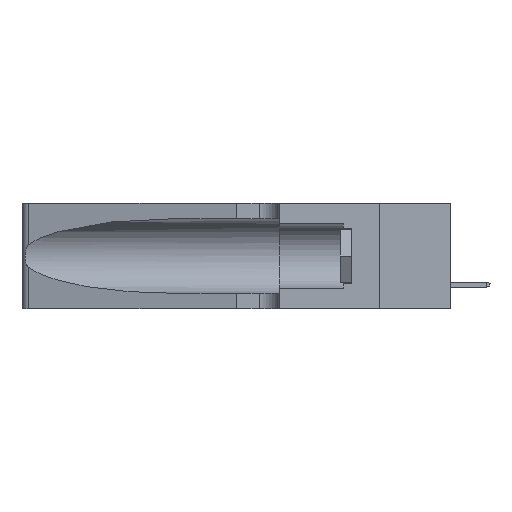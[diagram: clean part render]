
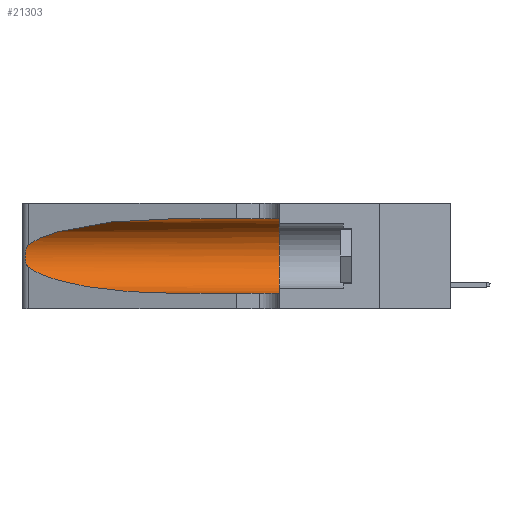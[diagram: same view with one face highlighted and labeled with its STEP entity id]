
A CAD part, left-side view. The second image highlights one B-rep face of the part: STEP entity #21303.
In plain terms, the highlighted cylindrical face has radius 3.308 mm (diameter 6.617 mm), a partial arc.
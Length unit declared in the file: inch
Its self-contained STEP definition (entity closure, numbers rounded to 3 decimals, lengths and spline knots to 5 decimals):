
#295 = CARTESIAN_POINT ( 'NONE',  ( 0.1305, 1.61858, 0.31525 ) ) ;
#780 = ORIENTED_EDGE ( 'NONE', *, *, #6802, .T. ) ;
#919 = CARTESIAN_POINT ( 'NONE',  ( 0.1305, 0.35, 0.05475 ) ) ;
#1037 = CARTESIAN_POINT ( 'NONE',  ( 0.25789, 1.23486, 0.15765 ) ) ;
#1840 = DIRECTION ( 'NONE',  ( 0., 0., 1. ) ) ;
#1937 = FACE_OUTER_BOUND ( 'NONE', #20477, .T. ) ;
#2094 = CARTESIAN_POINT ( 'NONE',  ( 0.1305, 0.72297, 0.31525 ) ) ;
#2103 = EDGE_CURVE ( 'NONE', #23419, #8402, #5209, .T. ) ;
#2304 = ORIENTED_EDGE ( 'NONE', *, *, #7361, .F. ) ;
#2541 = DIRECTION ( 'NONE',  ( 0., -1., 0. ) ) ;
#2750 = CARTESIAN_POINT ( 'NONE',  ( 0.25487, 1.22718, 0.22369 ) ) ;
#2828 = CARTESIAN_POINT ( 'NONE',  ( 0.2373, 1.15595, 0.08982 ) ) ;
#2834 = CARTESIAN_POINT ( 'NONE',  ( 0.1305, 1.61858, 0.185 ) ) ;
#3981 = CARTESIAN_POINT ( 'NONE',  ( 0.25854, 1.2359, 0.20912 ) ) ;
#5209 =( BOUNDED_CURVE ( )  B_SPLINE_CURVE ( 3, ( #16212, #23815, #19176, #16680 ),
 .UNSPECIFIED., .F., .F. ) 
 B_SPLINE_CURVE_WITH_KNOTS ( ( 4, 4 ),
 ( 1.5708, 2.84003 ),
 .UNSPECIFIED. ) 
 CURVE ( )  GEOMETRIC_REPRESENTATION_ITEM ( )  RATIONAL_B_SPLINE_CURVE ( ( 1., 0.87, 0.87, 1. ) ) 
 REPRESENTATION_ITEM ( '' )  );
#5874 = AXIS2_PLACEMENT_3D ( 'NONE', #23196, #6335, #1840 ) ;
#6311 = CARTESIAN_POINT ( 'NONE',  ( 0.25487, 1.22718, 0.14631 ) ) ;
#6335 = DIRECTION ( 'NONE',  ( 0., 1., 0. ) ) ;
#6802 = EDGE_CURVE ( 'NONE', #17899, #26115, #20473, .T. ) ;
#7361 = EDGE_CURVE ( 'NONE', #9910, #26115, #19382, .T. ) ;
#7679 = CARTESIAN_POINT ( 'NONE',  ( 0.1305, 0.72297, 0.05475 ) ) ;
#7943 = DIRECTION ( 'NONE',  ( 0., -1., 0. ) ) ;
#8219 =( BOUNDED_CURVE ( )  B_SPLINE_CURVE ( 3, ( #19090, #2828, #17208, #26074 ),
 .UNSPECIFIED., .F., .F. ) 
 B_SPLINE_CURVE_WITH_KNOTS ( ( 4, 4 ),
 ( 3.44316, 4.71239 ),
 .UNSPECIFIED. ) 
 CURVE ( )  GEOMETRIC_REPRESENTATION_ITEM ( )  RATIONAL_B_SPLINE_CURVE ( ( 1., 0.87, 0.87, 1. ) ) 
 REPRESENTATION_ITEM ( '' )  );
#8402 = VERTEX_POINT ( 'NONE', #29246 ) ;
#8641 = CARTESIAN_POINT ( 'NONE',  ( 0.25639, 1.23184, 0.21858 ) ) ;
#9910 = VERTEX_POINT ( 'NONE', #26938 ) ;
#10529 = CARTESIAN_POINT ( 'NONE',  ( 0.25555, 1.22994, 0.2215 ) ) ;
#10692 = CARTESIAN_POINT ( 'NONE',  ( 0.25639, 1.23186, 0.15144 ) ) ;
#11442 = CYLINDRICAL_SURFACE ( 'NONE', #19311, 0.13025 ) ;
#11825 = ORIENTED_EDGE ( 'NONE', *, *, #29089, .T. ) ;
#12564 = LINE ( 'NONE', #295, #20222 ) ;
#13182 = CARTESIAN_POINT ( 'NONE',  ( 0.26018, 1.23835, 0.19895 ) ) ;
#13494 = CARTESIAN_POINT ( 'NONE',  ( 0.26017, 1.23833, 0.17102 ) ) ;
#13564 = CARTESIAN_POINT ( 'NONE',  ( 0.25487, 1.22718, 0.14631 ) ) ;
#16190 = EDGE_CURVE ( 'NONE', #23419, #9910, #12564, .T. ) ;
#16212 = CARTESIAN_POINT ( 'NONE',  ( 0.1305, 0.72297, 0.31525 ) ) ;
#16680 = CARTESIAN_POINT ( 'NONE',  ( 0.25487, 1.22718, 0.22369 ) ) ;
#16853 = DIRECTION ( 'NONE',  ( 0., -1., 0. ) ) ;
#17208 = CARTESIAN_POINT ( 'NONE',  ( 0.18966, 0.96281, 0.05475 ) ) ;
#17231 = ORIENTED_EDGE ( 'NONE', *, *, #29840, .T. ) ;
#17899 = VERTEX_POINT ( 'NONE', #7679 ) ;
#18220 = CARTESIAN_POINT ( 'NONE',  ( 0.25856, 1.23593, 0.16098 ) ) ;
#18321 = VECTOR ( 'NONE', #7943, 39.37008 ) ;
#18434 = VERTEX_POINT ( 'NONE', #13564 ) ;
#19090 = CARTESIAN_POINT ( 'NONE',  ( 0.25487, 1.22718, 0.14631 ) ) ;
#19176 = CARTESIAN_POINT ( 'NONE',  ( 0.2373, 1.15595, 0.28018 ) ) ;
#19311 = AXIS2_PLACEMENT_3D ( 'NONE', #2834, #2541, #22034 ) ;
#19382 = CIRCLE ( 'NONE', #5874, 0.13025 ) ;
#20222 = VECTOR ( 'NONE', #16853, 39.37008 ) ;
#20473 = LINE ( 'NONE', #29926, #18321 ) ;
#20477 = EDGE_LOOP ( 'NONE', ( #26448, #11825, #17231, #780, #2304, #23935 ) ) ;
#21303 = ADVANCED_FACE ( 'NONE', ( #1937 ), #11442, .F. ) ;
#22034 = DIRECTION ( 'NONE',  ( 0., 0., -1. ) ) ;
#23196 = CARTESIAN_POINT ( 'NONE',  ( 0.1305, 0.35, 0.185 ) ) ;
#23419 = VERTEX_POINT ( 'NONE', #2094 ) ;
#23815 = CARTESIAN_POINT ( 'NONE',  ( 0.18966, 0.96281, 0.31525 ) ) ;
#23935 = ORIENTED_EDGE ( 'NONE', *, *, #16190, .F. ) ;
#24892 = CARTESIAN_POINT ( 'NONE',  ( 0.25555, 1.22993, 0.14849 ) ) ;
#25029 = CARTESIAN_POINT ( 'NONE',  ( 0.25787, 1.23484, 0.2124 ) ) ;
#25314 = B_SPLINE_CURVE_WITH_KNOTS ( 'NONE', 3,
 ( #2750, #10529, #8641, #25029, #3981, #13182, #27528, #27697, #13494, #18220, #1037, #10692, #24892, #6311 ),
 .UNSPECIFIED., .F., .F.,
 ( 4, 2, 2, 2, 2, 2, 4 ),
 ( 0., 0.00027, 0.00053, 0.00107, 0.0016, 0.00187, 0.00214 ),
 .UNSPECIFIED. ) ;
#26074 = CARTESIAN_POINT ( 'NONE',  ( 0.1305, 0.72297, 0.05475 ) ) ;
#26115 = VERTEX_POINT ( 'NONE', #919 ) ;
#26448 = ORIENTED_EDGE ( 'NONE', *, *, #2103, .T. ) ;
#26938 = CARTESIAN_POINT ( 'NONE',  ( 0.1305, 0.35, 0.31525 ) ) ;
#27528 = CARTESIAN_POINT ( 'NONE',  ( 0.26075, 1.23896, 0.19203 ) ) ;
#27697 = CARTESIAN_POINT ( 'NONE',  ( 0.26075, 1.23896, 0.178 ) ) ;
#29089 = EDGE_CURVE ( 'NONE', #8402, #18434, #25314, .T. ) ;
#29246 = CARTESIAN_POINT ( 'NONE',  ( 0.25487, 1.22718, 0.22369 ) ) ;
#29840 = EDGE_CURVE ( 'NONE', #18434, #17899, #8219, .T. ) ;
#29926 = CARTESIAN_POINT ( 'NONE',  ( 0.1305, 1.61858, 0.05475 ) ) ;
